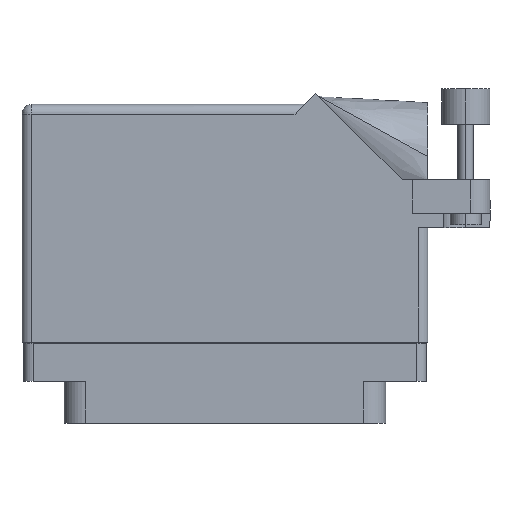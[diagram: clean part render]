
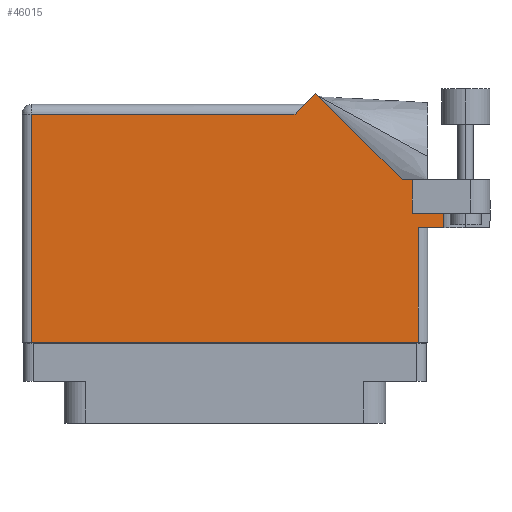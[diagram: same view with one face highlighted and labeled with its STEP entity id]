
A CAD part, front view. The second image highlights one B-rep face of the part: STEP entity #46015.
In plain terms, the highlighted face is planar.
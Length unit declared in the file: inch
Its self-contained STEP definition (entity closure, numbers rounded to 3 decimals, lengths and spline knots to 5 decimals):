
#128 = CARTESIAN_POINT ( 'NONE',  ( 1.244, -0.1, 0.455 ) ) ;
#713 = EDGE_CURVE ( 'NONE', #12408, #29481, #8407, .T. ) ;
#3151 = AXIS2_PLACEMENT_3D ( 'NONE', #12020, #12185, #41688 ) ;
#3289 = VERTEX_POINT ( 'NONE', #7130 ) ;
#4146 = VECTOR ( 'NONE', #9289, 39.37008 ) ;
#4434 = CARTESIAN_POINT ( 'NONE',  ( 1.14042, 0.944, 0.455 ) ) ;
#4460 = CARTESIAN_POINT ( 'NONE',  ( 1.206, 0.944, 0.455 ) ) ;
#4758 = DIRECTION ( 'NONE',  ( -0.707, -0.707, 0. ) ) ;
#4840 = ORIENTED_EDGE ( 'NONE', *, *, #12779, .F. ) ;
#5101 = VERTEX_POINT ( 'NONE', #40161 ) ;
#5921 = CARTESIAN_POINT ( 'NONE',  ( -1.244, -0.1, 0.455 ) ) ;
#7130 = CARTESIAN_POINT ( 'NONE',  ( 1.206, 0.731, 0.455 ) ) ;
#7506 = VERTEX_POINT ( 'NONE', #128 ) ;
#7776 = DIRECTION ( 'NONE',  ( 0., -1., 0. ) ) ;
#7954 = ORIENTED_EDGE ( 'NONE', *, *, #26873, .T. ) ;
#8407 = LINE ( 'NONE', #35802, #46443 ) ;
#8621 = LINE ( 'NONE', #4434, #9776 ) ;
#8813 = PLANE ( 'NONE',  #3151 ) ;
#9157 = LINE ( 'NONE', #27723, #42036 ) ;
#9289 = DIRECTION ( 'NONE',  ( -1., 0., 0. ) ) ;
#9555 = VECTOR ( 'NONE', #17048, 39.37008 ) ;
#9776 = VECTOR ( 'NONE', #34077, 39.37008 ) ;
#10499 = DIRECTION ( 'NONE',  ( 0., -1., 0. ) ) ;
#11174 = EDGE_CURVE ( 'NONE', #23944, #19433, #33566, .T. ) ;
#11417 = DIRECTION ( 'NONE',  ( -1., 0., 0. ) ) ;
#11813 = ORIENTED_EDGE ( 'NONE', *, *, #713, .T. ) ;
#12020 = CARTESIAN_POINT ( 'NONE',  ( -1.306, 1.43, 0.455 ) ) ;
#12091 = ORIENTED_EDGE ( 'NONE', *, *, #37473, .T. ) ;
#12185 = DIRECTION ( 'NONE',  ( 0., 0., -1. ) ) ;
#12290 = EDGE_CURVE ( 'NONE', #43836, #35227, #25396, .T. ) ;
#12326 = EDGE_CURVE ( 'NONE', #19114, #43836, #8621, .T. ) ;
#12408 = VERTEX_POINT ( 'NONE', #38422 ) ;
#12779 = EDGE_CURVE ( 'NONE', #5101, #19433, #33916, .T. ) ;
#13150 = EDGE_LOOP ( 'NONE', ( #7954, #12091, #46199, #4840, #37804, #23811, #33725, #21477, #27712, #18097, #11813 ) ) ;
#13378 = VECTOR ( 'NONE', #39678, 39.37008 ) ;
#15113 = LINE ( 'NONE', #28072, #13378 ) ;
#17048 = DIRECTION ( 'NONE',  ( 0., 1., 0. ) ) ;
#18097 = ORIENTED_EDGE ( 'NONE', *, *, #46934, .T. ) ;
#18726 = CARTESIAN_POINT ( 'NONE',  ( 1.4075, 1.06177, 0.455 ) ) ;
#19114 = VERTEX_POINT ( 'NONE', #31470 ) ;
#19272 = CARTESIAN_POINT ( 'NONE',  ( 0.513, 1.43, 0.455 ) ) ;
#19433 = VERTEX_POINT ( 'NONE', #40531 ) ;
#21477 = ORIENTED_EDGE ( 'NONE', *, *, #12326, .T. ) ;
#22421 = CARTESIAN_POINT ( 'NONE',  ( 0.58371, 1.50071, 0.455 ) ) ;
#22594 = VECTOR ( 'NONE', #31476, 39.37008 ) ;
#23050 = CARTESIAN_POINT ( 'NONE',  ( 1.244, 0.637, 0.455 ) ) ;
#23676 = CARTESIAN_POINT ( 'NONE',  ( 1.206, 0.731, 0.455 ) ) ;
#23811 = ORIENTED_EDGE ( 'NONE', *, *, #25678, .T. ) ;
#23944 = VERTEX_POINT ( 'NONE', #23050 ) ;
#24015 = VECTOR ( 'NONE', #26463, 39.37008 ) ;
#25396 = LINE ( 'NONE', #19272, #46101 ) ;
#25678 = EDGE_CURVE ( 'NONE', #3289, #38604, #34943, .T. ) ;
#26116 = CARTESIAN_POINT ( 'NONE',  ( -1.306, 1.368, 0.455 ) ) ;
#26463 = DIRECTION ( 'NONE',  ( 1., 0., 0. ) ) ;
#26873 = EDGE_CURVE ( 'NONE', #29481, #7506, #15113, .T. ) ;
#27712 = ORIENTED_EDGE ( 'NONE', *, *, #12290, .T. ) ;
#27723 = CARTESIAN_POINT ( 'NONE',  ( 1.244, 0.637, 0.455 ) ) ;
#28067 = EDGE_CURVE ( 'NONE', #3289, #5101, #29714, .T. ) ;
#28072 = CARTESIAN_POINT ( 'NONE',  ( -1.306, -0.1, 0.455 ) ) ;
#29481 = VERTEX_POINT ( 'NONE', #5921 ) ;
#29494 = CARTESIAN_POINT ( 'NONE',  ( 1.206, 0.731, 0.455 ) ) ;
#29714 = LINE ( 'NONE', #29494, #24015 ) ;
#31247 = DIRECTION ( 'NONE',  ( 0., 1., 0. ) ) ;
#31470 = CARTESIAN_POINT ( 'NONE',  ( 1.14042, 0.944, 0.455 ) ) ;
#31476 = DIRECTION ( 'NONE',  ( 1., 0., 0. ) ) ;
#31804 = CARTESIAN_POINT ( 'NONE',  ( 1.306, 0.637, 0.455 ) ) ;
#33566 = LINE ( 'NONE', #31804, #22594 ) ;
#33725 = ORIENTED_EDGE ( 'NONE', *, *, #47539, .T. ) ;
#33916 = LINE ( 'NONE', #18726, #37988 ) ;
#34077 = DIRECTION ( 'NONE',  ( -0.707, 0.707, 0. ) ) ;
#34943 = LINE ( 'NONE', #23676, #9555 ) ;
#35227 = VERTEX_POINT ( 'NONE', #37720 ) ;
#35802 = CARTESIAN_POINT ( 'NONE',  ( -1.244, -0.1, 0.455 ) ) ;
#37207 = FACE_OUTER_BOUND ( 'NONE', #13150, .T. ) ;
#37473 = EDGE_CURVE ( 'NONE', #7506, #23944, #9157, .T. ) ;
#37720 = CARTESIAN_POINT ( 'NONE',  ( 0.451, 1.368, 0.455 ) ) ;
#37804 = ORIENTED_EDGE ( 'NONE', *, *, #28067, .F. ) ;
#37988 = VECTOR ( 'NONE', #7776, 39.37008 ) ;
#37990 = CARTESIAN_POINT ( 'NONE',  ( 1.706, 0.944, 0.455 ) ) ;
#38422 = CARTESIAN_POINT ( 'NONE',  ( -1.244, 1.368, 0.455 ) ) ;
#38604 = VERTEX_POINT ( 'NONE', #4460 ) ;
#39678 = DIRECTION ( 'NONE',  ( 1., 0., 0. ) ) ;
#40161 = CARTESIAN_POINT ( 'NONE',  ( 1.4075, 0.731, 0.455 ) ) ;
#40531 = CARTESIAN_POINT ( 'NONE',  ( 1.4075, 0.637, 0.455 ) ) ;
#40591 = VECTOR ( 'NONE', #11417, 39.37008 ) ;
#41065 = LINE ( 'NONE', #37990, #4146 ) ;
#41688 = DIRECTION ( 'NONE',  ( -1., 0., 0. ) ) ;
#42036 = VECTOR ( 'NONE', #31247, 39.37008 ) ;
#43836 = VERTEX_POINT ( 'NONE', #22421 ) ;
#46015 = ADVANCED_FACE ( 'NONE', ( #37207 ), #8813, .F. ) ;
#46101 = VECTOR ( 'NONE', #4758, 39.37008 ) ;
#46199 = ORIENTED_EDGE ( 'NONE', *, *, #11174, .T. ) ;
#46443 = VECTOR ( 'NONE', #10499, 39.37008 ) ;
#46860 = LINE ( 'NONE', #26116, #40591 ) ;
#46934 = EDGE_CURVE ( 'NONE', #35227, #12408, #46860, .T. ) ;
#47539 = EDGE_CURVE ( 'NONE', #38604, #19114, #41065, .T. ) ;
